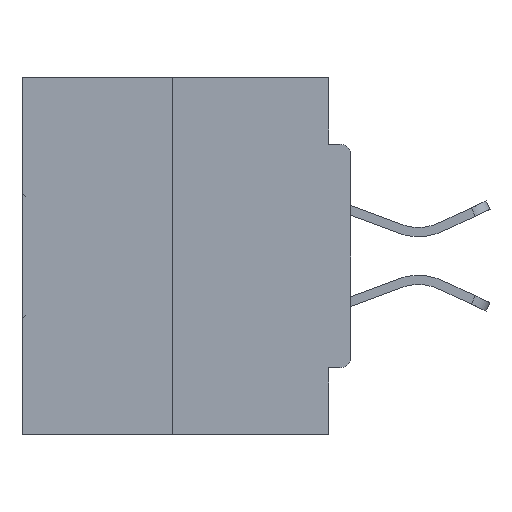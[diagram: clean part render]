
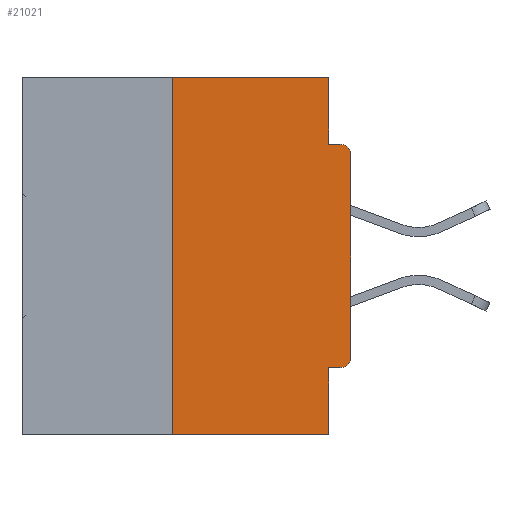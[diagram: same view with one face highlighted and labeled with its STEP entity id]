
A CAD part, left-side view. The second image highlights one B-rep face of the part: STEP entity #21021.
In plain terms, the highlighted planar face has unit normal (-1, 0, 0).
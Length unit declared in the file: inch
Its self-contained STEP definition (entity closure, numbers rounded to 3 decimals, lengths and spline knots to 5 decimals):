
#147 = DIRECTION ( 'NONE',  ( 0., 0., -1. ) ) ;
#295 = VERTEX_POINT ( 'NONE', #40162 ) ;
#1388 = DIRECTION ( 'NONE',  ( 0., -1., 0. ) ) ;
#1920 = EDGE_CURVE ( 'NONE', #17863, #33200, #33327, .T. ) ;
#2147 = LINE ( 'NONE', #22430, #28789 ) ;
#2404 = ORIENTED_EDGE ( 'NONE', *, *, #24975, .F. ) ;
#2422 = DIRECTION ( 'NONE',  ( 0., 0., 1. ) ) ;
#3922 = CARTESIAN_POINT ( 'NONE',  ( 0., 0.015, -0.3915 ) ) ;
#4014 = EDGE_CURVE ( 'NONE', #21640, #21412, #33478, .T. ) ;
#4096 = LINE ( 'NONE', #39583, #9799 ) ;
#5519 = CARTESIAN_POINT ( 'NONE',  ( 0., 0.031, 0. ) ) ;
#5708 = CARTESIAN_POINT ( 'NONE',  ( 0., 0., -0.4065 ) ) ;
#5914 = DIRECTION ( 'NONE',  ( 0., 0., 1. ) ) ;
#6283 = FACE_OUTER_BOUND ( 'NONE', #9413, .T. ) ;
#6343 = CARTESIAN_POINT ( 'NONE',  ( 0., 0.031, -0.4065 ) ) ;
#6713 = EDGE_CURVE ( 'NONE', #295, #21412, #23907, .T. ) ;
#7336 = AXIS2_PLACEMENT_3D ( 'NONE', #3922, #13561, #147 ) ;
#8005 = CARTESIAN_POINT ( 'NONE',  ( 0., 0.031, -0.5 ) ) ;
#8443 = DIRECTION ( 'NONE',  ( 0., 1., 0. ) ) ;
#8846 = DIRECTION ( 'NONE',  ( 0., 0., -1. ) ) ;
#9393 = CARTESIAN_POINT ( 'NONE',  ( 0., 0.46, 0. ) ) ;
#9413 = EDGE_LOOP ( 'NONE', ( #26148, #35559, #11012, #12566, #2404, #41126, #22825, #10836, #18606, #17115 ) ) ;
#9799 = VECTOR ( 'NONE', #2422, 39.37008 ) ;
#9820 = CARTESIAN_POINT ( 'NONE',  ( 0., 0.015, -0.1085 ) ) ;
#10836 = ORIENTED_EDGE ( 'NONE', *, *, #1920, .T. ) ;
#11012 = ORIENTED_EDGE ( 'NONE', *, *, #6713, .T. ) ;
#11040 = EDGE_CURVE ( 'NONE', #20949, #38513, #11461, .T. ) ;
#11461 = LINE ( 'NONE', #5519, #25045 ) ;
#12566 = ORIENTED_EDGE ( 'NONE', *, *, #4014, .F. ) ;
#12582 = VECTOR ( 'NONE', #34789, 39.37008 ) ;
#12685 = EDGE_CURVE ( 'NONE', #26526, #27431, #35840, .T. ) ;
#12918 = DIRECTION ( 'NONE',  ( 0., 0., -1. ) ) ;
#13561 = DIRECTION ( 'NONE',  ( -1., 0., 0. ) ) ;
#13985 = VECTOR ( 'NONE', #23365, 39.37008 ) ;
#15920 = EDGE_CURVE ( 'NONE', #19857, #20949, #21909, .T. ) ;
#17101 = VECTOR ( 'NONE', #8443, 39.37008 ) ;
#17115 = ORIENTED_EDGE ( 'NONE', *, *, #11040, .F. ) ;
#17747 = CARTESIAN_POINT ( 'NONE',  ( 0., 0., -0.1085 ) ) ;
#17863 = VERTEX_POINT ( 'NONE', #17747 ) ;
#18606 = ORIENTED_EDGE ( 'NONE', *, *, #30217, .F. ) ;
#19569 = CARTESIAN_POINT ( 'NONE',  ( 0., 0., -0.0935 ) ) ;
#19857 = VERTEX_POINT ( 'NONE', #24694 ) ;
#20949 = VERTEX_POINT ( 'NONE', #38886 ) ;
#21021 = ADVANCED_FACE ( 'NONE', ( #6283 ), #39729, .F. ) ;
#21049 = CARTESIAN_POINT ( 'NONE',  ( 0., 0.015, -0.0935 ) ) ;
#21412 = VERTEX_POINT ( 'NONE', #8005 ) ;
#21640 = VERTEX_POINT ( 'NONE', #6343 ) ;
#21909 = LINE ( 'NONE', #37851, #32325 ) ;
#22430 = CARTESIAN_POINT ( 'NONE',  ( 0., 0.25, 0. ) ) ;
#22714 = DIRECTION ( 'NONE',  ( 0., 0., -1. ) ) ;
#22825 = ORIENTED_EDGE ( 'NONE', *, *, #23458, .T. ) ;
#23006 = DIRECTION ( 'NONE',  ( -1., 0., 0. ) ) ;
#23365 = DIRECTION ( 'NONE',  ( 0., -1., 0. ) ) ;
#23458 = EDGE_CURVE ( 'NONE', #27431, #17863, #4096, .T. ) ;
#23656 = CARTESIAN_POINT ( 'NONE',  ( 0., 0., -0.3915 ) ) ;
#23907 = LINE ( 'NONE', #33540, #13985 ) ;
#24439 = CARTESIAN_POINT ( 'NONE',  ( 0., 0.031, -0.5 ) ) ;
#24694 = CARTESIAN_POINT ( 'NONE',  ( 0., 0.25, 0. ) ) ;
#24975 = EDGE_CURVE ( 'NONE', #26526, #21640, #37969, .T. ) ;
#25045 = VECTOR ( 'NONE', #8846, 39.37008 ) ;
#26024 = AXIS2_PLACEMENT_3D ( 'NONE', #9393, #32770, #22714 ) ;
#26148 = ORIENTED_EDGE ( 'NONE', *, *, #15920, .F. ) ;
#26526 = VERTEX_POINT ( 'NONE', #33887 ) ;
#27287 = LINE ( 'NONE', #19569, #38751 ) ;
#27431 = VERTEX_POINT ( 'NONE', #23656 ) ;
#28789 = VECTOR ( 'NONE', #5914, 39.37008 ) ;
#29777 = DIRECTION ( 'NONE',  ( 0., -1., 0. ) ) ;
#30217 = EDGE_CURVE ( 'NONE', #38513, #33200, #27287, .T. ) ;
#31187 = EDGE_CURVE ( 'NONE', #295, #19857, #2147, .T. ) ;
#32325 = VECTOR ( 'NONE', #1388, 39.37008 ) ;
#32770 = DIRECTION ( 'NONE',  ( 1., 0., 0. ) ) ;
#33200 = VERTEX_POINT ( 'NONE', #21049 ) ;
#33327 = CIRCLE ( 'NONE', #39094, 0.015 ) ;
#33432 = CARTESIAN_POINT ( 'NONE',  ( 0., 0.031, -0.0935 ) ) ;
#33478 = LINE ( 'NONE', #24439, #12582 ) ;
#33540 = CARTESIAN_POINT ( 'NONE',  ( 0., 0.46, -0.5 ) ) ;
#33887 = CARTESIAN_POINT ( 'NONE',  ( 0., 0.015, -0.4065 ) ) ;
#34789 = DIRECTION ( 'NONE',  ( 0., 0., -1. ) ) ;
#35559 = ORIENTED_EDGE ( 'NONE', *, *, #31187, .F. ) ;
#35840 = CIRCLE ( 'NONE', #7336, 0.015 ) ;
#37851 = CARTESIAN_POINT ( 'NONE',  ( 0., 0.46, 0. ) ) ;
#37969 = LINE ( 'NONE', #5708, #17101 ) ;
#38513 = VERTEX_POINT ( 'NONE', #33432 ) ;
#38751 = VECTOR ( 'NONE', #29777, 39.37008 ) ;
#38886 = CARTESIAN_POINT ( 'NONE',  ( 0., 0.031, 0. ) ) ;
#39094 = AXIS2_PLACEMENT_3D ( 'NONE', #9820, #23006, #12918 ) ;
#39583 = CARTESIAN_POINT ( 'NONE',  ( 0., 0., 0. ) ) ;
#39729 = PLANE ( 'NONE',  #26024 ) ;
#40162 = CARTESIAN_POINT ( 'NONE',  ( 0., 0.25, -0.5 ) ) ;
#41126 = ORIENTED_EDGE ( 'NONE', *, *, #12685, .T. ) ;
